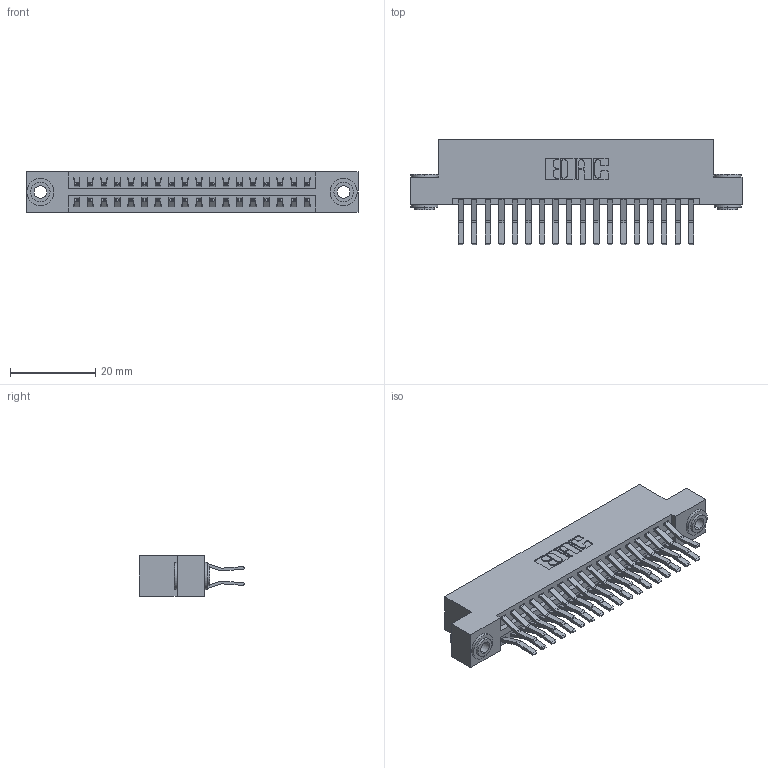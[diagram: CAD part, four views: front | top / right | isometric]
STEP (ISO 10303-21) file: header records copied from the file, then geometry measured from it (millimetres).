
FILE_DESCRIPTION (( 'STEP AP203' ), '1' );
FILE_NAME ('346-036-560-203.STEP', '2022-05-19T22:36:53', ( '' ), ( '' ), 'SwSTEP 2.0', 'SolidWorks 2020', '' );
FILE_SCHEMA (( 'CONFIG_CONTROL_DESIGN' ));
Length unit declared in the file: inch
Products named in the file (4): 346-036-560-203; 346 Part_Flush Mounting Lugs - 0.156 Dia-TH; 345-250-002_345-250-002-102; 345-292-001_560 Tail
Assembly tree (39 placements, depth 2):
  346-036-560-203
    346 Part_Flush Mounting Lugs - 0.156 Dia-TH
    345-292-001_560 Tail  x36
    345-250-002_345-250-002-102  x2
Bounding box: 77.72 x 24.78 x 9.4 mm (x, y, z)
Volume: 7629.9 mm3; surface area: 10988.9 mm2
Topology: 39 solids, 39 shells, 2118 faces, 6237 edges, 4106 vertices
Faces by surface type: plane 1360, cylinder 750, cone 8
Entity records: 16132 total; most frequent: CARTESIAN_POINT 2673, ORIENTED_EDGE 2598, DIRECTION 2441, EDGE_CURVE 1299, VECTOR 1067, LINE 1067, VERTEX_POINT 862, AXIS2_PLACEMENT_3D 687
